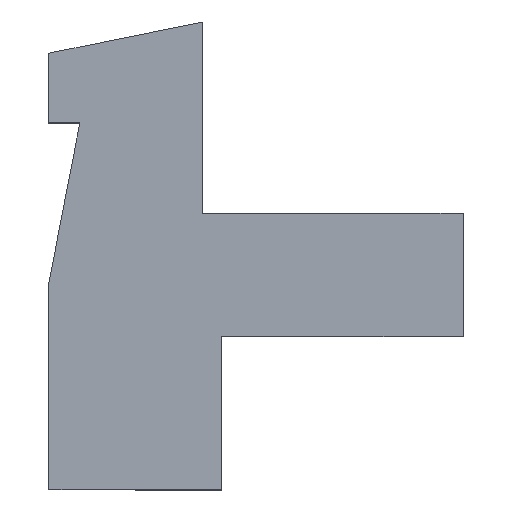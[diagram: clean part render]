
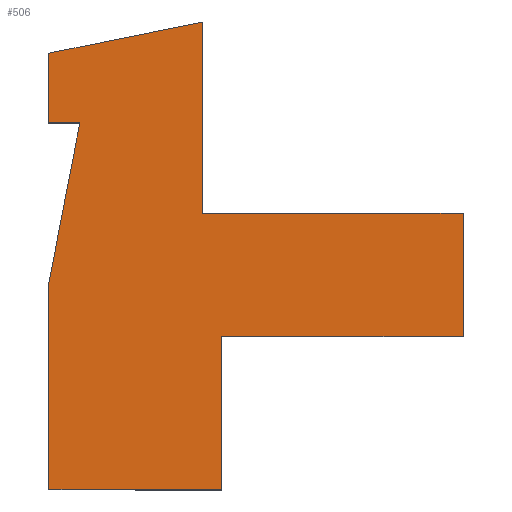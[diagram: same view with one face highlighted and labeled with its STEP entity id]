
A CAD part, top view. The second image highlights one B-rep face of the part: STEP entity #506.
In plain terms, the highlighted planar face has unit normal (0, 0, 1).
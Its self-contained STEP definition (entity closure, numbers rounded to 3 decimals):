
#11 = FACE_OUTER_BOUND ( 'NONE', #54, .T. ) ;
#14 = VERTEX_POINT ( 'NONE', #52 ) ;
#27 = VERTEX_POINT ( 'NONE', #159 ) ;
#29 = DIRECTION ( 'NONE',  ( 0., -1., 0. ) ) ;
#30 = CARTESIAN_POINT ( 'NONE',  ( -25.337, 8.542, 6. ) ) ;
#34 = ORIENTED_EDGE ( 'NONE', *, *, #648, .T. ) ;
#45 = EDGE_CURVE ( 'NONE', #488, #14, #55, .T. ) ;
#49 = CARTESIAN_POINT ( 'NONE',  ( -27.325, 1.586, 6. ) ) ;
#52 = CARTESIAN_POINT ( 'NONE',  ( -25.337, 3.339, 6. ) ) ;
#54 = EDGE_LOOP ( 'NONE', ( #689, #177, #314, #590, #519, #456, #352, #322, #34, #649, #587, #137, #452, #423 ) ) ;
#55 = LINE ( 'NONE', #164, #499 ) ;
#57 = VERTEX_POINT ( 'NONE', #603 ) ;
#62 = AXIS2_PLACEMENT_3D ( 'NONE', #658, #602, #292 ) ;
#75 = CARTESIAN_POINT ( 'NONE',  ( -19.7, -3.414, 6. ) ) ;
#83 = CARTESIAN_POINT ( 'NONE',  ( -24.498, 7.643, 6. ) ) ;
#84 = DIRECTION ( 'NONE',  ( 0., 1., 0. ) ) ;
#122 = DIRECTION ( 'NONE',  ( 0., -1., 0. ) ) ;
#126 = EDGE_CURVE ( 'NONE', #341, #478, #659, .T. ) ;
#128 = CARTESIAN_POINT ( 'NONE',  ( -25.337, 10.807, 6. ) ) ;
#133 = CARTESIAN_POINT ( 'NONE',  ( -19.7, -32.29, 6. ) ) ;
#137 = ORIENTED_EDGE ( 'NONE', *, *, #481, .T. ) ;
#147 = CARTESIAN_POINT ( 'NONE',  ( -25.337, -3.414, 6. ) ) ;
#157 = VERTEX_POINT ( 'NONE', #269 ) ;
#159 = CARTESIAN_POINT ( 'NONE',  ( -11.837, 5.586, 6. ) ) ;
#164 = CARTESIAN_POINT ( 'NONE',  ( -24.326, 8.542, 6. ) ) ;
#172 = VECTOR ( 'NONE', #122, 1000. ) ;
#177 = ORIENTED_EDGE ( 'NONE', *, *, #309, .F. ) ;
#178 = DIRECTION ( 'NONE',  ( 1., 0., 0. ) ) ;
#182 = CARTESIAN_POINT ( 'NONE',  ( -24.498, 7.643, 6. ) ) ;
#184 = VERTEX_POINT ( 'NONE', #546 ) ;
#185 = DIRECTION ( 'NONE',  ( 1., 0., 0. ) ) ;
#209 = EDGE_CURVE ( 'NONE', #27, #184, #492, .T. ) ;
#212 = VECTOR ( 'NONE', #595, 1000. ) ;
#229 = EDGE_CURVE ( 'NONE', #157, #27, #645, .T. ) ;
#246 = VECTOR ( 'NONE', #471, 1000. ) ;
#266 = EDGE_CURVE ( 'NONE', #524, #680, #297, .T. ) ;
#268 = LINE ( 'NONE', #336, #212 ) ;
#269 = CARTESIAN_POINT ( 'NONE',  ( -20.337, 5.586, 6. ) ) ;
#276 = CARTESIAN_POINT ( 'NONE',  ( -20.337, 5.586, 6. ) ) ;
#292 = DIRECTION ( 'NONE',  ( 1., 0., 0. ) ) ;
#294 = VECTOR ( 'NONE', #84, 1000. ) ;
#297 = LINE ( 'NONE', #569, #625 ) ;
#309 = EDGE_CURVE ( 'NONE', #570, #14, #512, .T. ) ;
#314 = ORIENTED_EDGE ( 'NONE', *, *, #462, .T. ) ;
#322 = ORIENTED_EDGE ( 'NONE', *, *, #615, .F. ) ;
#335 = VERTEX_POINT ( 'NONE', #508 ) ;
#336 = CARTESIAN_POINT ( 'NONE',  ( -24.326, 8.542, 6. ) ) ;
#339 = VECTOR ( 'NONE', #29, 1000. ) ;
#341 = VERTEX_POINT ( 'NONE', #30 ) ;
#343 = DIRECTION ( 'NONE',  ( 0., -1., 0. ) ) ;
#352 = ORIENTED_EDGE ( 'NONE', *, *, #229, .F. ) ;
#359 = CARTESIAN_POINT ( 'NONE',  ( -24.501, 7.643, 6. ) ) ;
#364 = EDGE_CURVE ( 'NONE', #524, #488, #663, .T. ) ;
#365 = EDGE_CURVE ( 'NONE', #594, #400, #611, .T. ) ;
#370 = DIRECTION ( 'NONE',  ( 1., 0., 0. ) ) ;
#375 = DIRECTION ( 'NONE',  ( 0., 1., 0. ) ) ;
#388 = LINE ( 'NONE', #653, #521 ) ;
#399 = DIRECTION ( 'NONE',  ( -0.193, -0.981, 0. ) ) ;
#400 = VERTEX_POINT ( 'NONE', #75 ) ;
#408 = VECTOR ( 'NONE', #185, 1000. ) ;
#419 = LINE ( 'NONE', #49, #567 ) ;
#423 = ORIENTED_EDGE ( 'NONE', *, *, #364, .T. ) ;
#426 = CARTESIAN_POINT ( 'NONE',  ( -11.837, -8.414, 6. ) ) ;
#443 = PLANE ( 'NONE',  #62 ) ;
#450 = CARTESIAN_POINT ( 'NONE',  ( -19.7, 1.586, 6. ) ) ;
#452 = ORIENTED_EDGE ( 'NONE', *, *, #266, .F. ) ;
#456 = ORIENTED_EDGE ( 'NONE', *, *, #209, .F. ) ;
#459 = DIRECTION ( 'NONE',  ( -1., 0., 0. ) ) ;
#462 = EDGE_CURVE ( 'NONE', #570, #400, #388, .T. ) ;
#466 = VECTOR ( 'NONE', #399, 1000. ) ;
#471 = DIRECTION ( 'NONE',  ( -0.98, -0.199, 0. ) ) ;
#478 = VERTEX_POINT ( 'NONE', #128 ) ;
#481 = EDGE_CURVE ( 'NONE', #335, #680, #268, .T. ) ;
#488 = VERTEX_POINT ( 'NONE', #541 ) ;
#492 = LINE ( 'NONE', #426, #172 ) ;
#499 = VECTOR ( 'NONE', #691, 1000. ) ;
#506 = ADVANCED_FACE ( 'NONE', ( #11 ), #443, .T. ) ;
#508 = CARTESIAN_POINT ( 'NONE',  ( -24.326, 8.542, 6. ) ) ;
#510 = LINE ( 'NONE', #668, #339 ) ;
#512 = LINE ( 'NONE', #516, #294 ) ;
#516 = CARTESIAN_POINT ( 'NONE',  ( -25.337, -8.414, 6. ) ) ;
#519 = ORIENTED_EDGE ( 'NONE', *, *, #688, .F. ) ;
#521 = VECTOR ( 'NONE', #178, 1000. ) ;
#524 = VERTEX_POINT ( 'NONE', #83 ) ;
#527 = CARTESIAN_POINT ( 'NONE',  ( -18.822, 12.133, 6. ) ) ;
#529 = VECTOR ( 'NONE', #370, 1000. ) ;
#536 = CARTESIAN_POINT ( 'NONE',  ( -25.337, -8.414, 6. ) ) ;
#541 = CARTESIAN_POINT ( 'NONE',  ( -24.719, 6.523, 6. ) ) ;
#546 = CARTESIAN_POINT ( 'NONE',  ( -11.837, 1.586, 6. ) ) ;
#558 = LINE ( 'NONE', #672, #408 ) ;
#567 = VECTOR ( 'NONE', #580, 1000. ) ;
#569 = CARTESIAN_POINT ( 'NONE',  ( -28.016, 7.643, 6. ) ) ;
#570 = VERTEX_POINT ( 'NONE', #147 ) ;
#580 = DIRECTION ( 'NONE',  ( -1., 0., 0. ) ) ;
#586 = VECTOR ( 'NONE', #343, 1000. ) ;
#587 = ORIENTED_EDGE ( 'NONE', *, *, #621, .T. ) ;
#590 = ORIENTED_EDGE ( 'NONE', *, *, #365, .F. ) ;
#594 = VERTEX_POINT ( 'NONE', #450 ) ;
#595 = DIRECTION ( 'NONE',  ( -0.191, -0.982, 0. ) ) ;
#602 = DIRECTION ( 'NONE',  ( 0., 0., 1. ) ) ;
#603 = CARTESIAN_POINT ( 'NONE',  ( -20.337, 11.825, 6. ) ) ;
#609 = VECTOR ( 'NONE', #375, 1000. ) ;
#611 = LINE ( 'NONE', #133, #586 ) ;
#615 = EDGE_CURVE ( 'NONE', #57, #157, #510, .T. ) ;
#621 = EDGE_CURVE ( 'NONE', #341, #335, #558, .T. ) ;
#625 = VECTOR ( 'NONE', #459, 1000. ) ;
#645 = LINE ( 'NONE', #276, #529 ) ;
#648 = EDGE_CURVE ( 'NONE', #57, #478, #686, .T. ) ;
#649 = ORIENTED_EDGE ( 'NONE', *, *, #126, .F. ) ;
#653 = CARTESIAN_POINT ( 'NONE',  ( -25.337, -3.414, 6. ) ) ;
#658 = CARTESIAN_POINT ( 'NONE',  ( -11.837, -8.414, 6. ) ) ;
#659 = LINE ( 'NONE', #536, #609 ) ;
#663 = LINE ( 'NONE', #182, #466 ) ;
#668 = CARTESIAN_POINT ( 'NONE',  ( -20.337, 12.086, 6. ) ) ;
#672 = CARTESIAN_POINT ( 'NONE',  ( -11.837, 8.542, 6. ) ) ;
#680 = VERTEX_POINT ( 'NONE', #359 ) ;
#686 = LINE ( 'NONE', #527, #246 ) ;
#688 = EDGE_CURVE ( 'NONE', #184, #594, #419, .T. ) ;
#689 = ORIENTED_EDGE ( 'NONE', *, *, #45, .T. ) ;
#691 = DIRECTION ( 'NONE',  ( -0.191, -0.982, 0. ) ) ;
